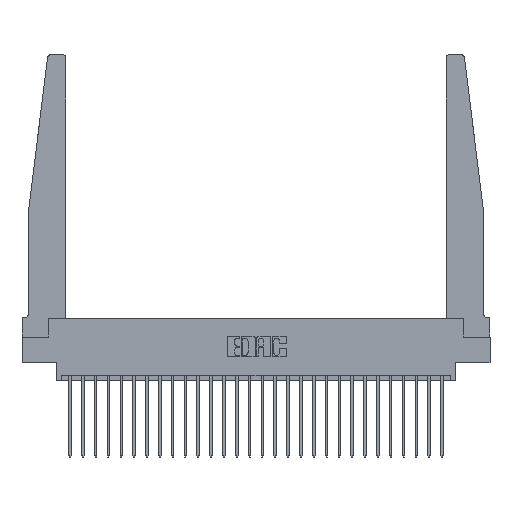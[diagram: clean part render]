
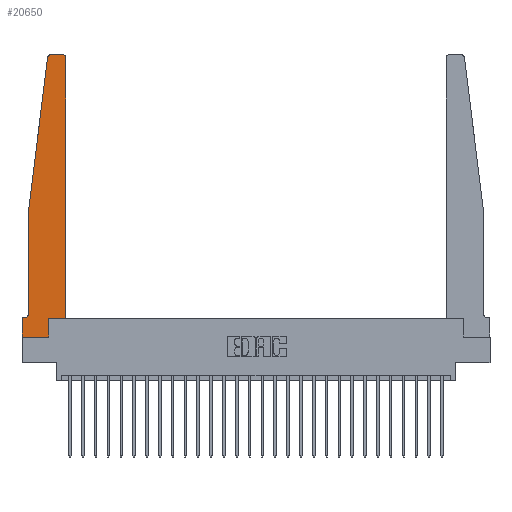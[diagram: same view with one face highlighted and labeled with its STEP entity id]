
A CAD part, top view. The second image highlights one B-rep face of the part: STEP entity #20650.
In plain terms, the highlighted planar face has unit normal (0, 0, 1).
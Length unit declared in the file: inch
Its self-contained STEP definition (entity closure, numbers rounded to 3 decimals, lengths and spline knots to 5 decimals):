
#593 = CARTESIAN_POINT ( 'NONE',  ( 0.395, 2.75, 0.37 ) ) ;
#656 = CARTESIAN_POINT ( 'NONE',  ( 0.2605, 0.18, 0.37 ) ) ;
#1507 = EDGE_LOOP ( 'NONE', ( #20498, #9159, #24146, #10517, #12868, #6242, #23240, #23998, #9563, #15301, #3218, #22295 ) ) ;
#1535 = VERTEX_POINT ( 'NONE', #5491 ) ;
#1877 = CARTESIAN_POINT ( 'NONE',  ( 0.065, 1.25, 0.37 ) ) ;
#2134 = EDGE_CURVE ( 'NONE', #16130, #18768, #19901, .T. ) ;
#2393 = DIRECTION ( 'NONE',  ( -1., 0., 0. ) ) ;
#2417 = CARTESIAN_POINT ( 'NONE',  ( 0.2605, 0.18, 0.37 ) ) ;
#2565 = AXIS2_PLACEMENT_3D ( 'NONE', #11643, #25686, #13702 ) ;
#2702 = EDGE_CURVE ( 'NONE', #18005, #11768, #7835, .T. ) ;
#2938 = AXIS2_PLACEMENT_3D ( 'NONE', #18687, #6571, #20726 ) ;
#3218 = ORIENTED_EDGE ( 'NONE', *, *, #19255, .T. ) ;
#3712 = VECTOR ( 'NONE', #24651, 39.37008 ) ;
#3942 = DIRECTION ( 'NONE',  ( 0., -1., 0. ) ) ;
#4295 = LINE ( 'NONE', #1877, #14464 ) ;
#4503 = CIRCLE ( 'NONE', #8227, 0.03 ) ;
#5489 = EDGE_CURVE ( 'NONE', #10939, #11011, #11783, .T. ) ;
#5491 = CARTESIAN_POINT ( 'NONE',  ( 0., 0., 0.37 ) ) ;
#5632 = CARTESIAN_POINT ( 'NONE',  ( 0.2605, 0., 0.37 ) ) ;
#6242 = ORIENTED_EDGE ( 'NONE', *, *, #2134, .T. ) ;
#6341 = EDGE_CURVE ( 'NONE', #15862, #16130, #15531, .T. ) ;
#6571 = DIRECTION ( 'NONE',  ( 0., 0., -1. ) ) ;
#6700 = DIRECTION ( 'NONE',  ( 1., 0., 0. ) ) ;
#7031 = VERTEX_POINT ( 'NONE', #2417 ) ;
#7835 = LINE ( 'NONE', #14583, #19243 ) ;
#8184 = AXIS2_PLACEMENT_3D ( 'NONE', #9942, #24029, #11977 ) ;
#8227 = AXIS2_PLACEMENT_3D ( 'NONE', #9074, #23188, #11116 ) ;
#8723 = LINE ( 'NONE', #24574, #23569 ) ;
#9074 = CARTESIAN_POINT ( 'NONE',  ( 0.27653, 2.72, 0.37 ) ) ;
#9159 = ORIENTED_EDGE ( 'NONE', *, *, #22400, .T. ) ;
#9563 = ORIENTED_EDGE ( 'NONE', *, *, #18704, .T. ) ;
#9791 = VECTOR ( 'NONE', #16907, 39.37008 ) ;
#9815 = CARTESIAN_POINT ( 'NONE',  ( 0.015, 0.1875, 0.37 ) ) ;
#9942 = CARTESIAN_POINT ( 'NONE',  ( 0.395, 2.72, 0.37 ) ) ;
#10312 = CARTESIAN_POINT ( 'NONE',  ( 0.24675, 2.72367, 0.37 ) ) ;
#10355 = DIRECTION ( 'NONE',  ( -1., 0., 0. ) ) ;
#10447 = VERTEX_POINT ( 'NONE', #5632 ) ;
#10517 = ORIENTED_EDGE ( 'NONE', *, *, #16203, .T. ) ;
#10580 = CARTESIAN_POINT ( 'NONE',  ( 0.425, 0.18, 0.37 ) ) ;
#10719 = CARTESIAN_POINT ( 'NONE',  ( 0.425, 0.18, 0.37 ) ) ;
#10727 = EDGE_CURVE ( 'NONE', #18768, #1535, #8723, .T. ) ;
#10743 = VECTOR ( 'NONE', #6700, 39.37008 ) ;
#10939 = VERTEX_POINT ( 'NONE', #10312 ) ;
#11011 = VERTEX_POINT ( 'NONE', #14552 ) ;
#11116 = DIRECTION ( 'NONE',  ( 1., 0., 0. ) ) ;
#11643 = CARTESIAN_POINT ( 'NONE',  ( 0., 0.1875, 0.37 ) ) ;
#11666 = DIRECTION ( 'NONE',  ( -0.122, -0.992, 0. ) ) ;
#11768 = VERTEX_POINT ( 'NONE', #12862 ) ;
#11783 = LINE ( 'NONE', #13730, #21899 ) ;
#11867 = EDGE_CURVE ( 'NONE', #7031, #25338, #25058, .T. ) ;
#11977 = DIRECTION ( 'NONE',  ( 1., 0., 0. ) ) ;
#12405 = CARTESIAN_POINT ( 'NONE',  ( 0.065, 0.1875, 0.37 ) ) ;
#12847 = VERTEX_POINT ( 'NONE', #16609 ) ;
#12862 = CARTESIAN_POINT ( 'NONE',  ( 0.27653, 2.75, 0.37 ) ) ;
#12868 = ORIENTED_EDGE ( 'NONE', *, *, #6341, .T. ) ;
#13219 = DIRECTION ( 'NONE',  ( 1., 0., 0. ) ) ;
#13702 = DIRECTION ( 'NONE',  ( 1., 0., 0. ) ) ;
#13730 = CARTESIAN_POINT ( 'NONE',  ( 0.065, 1.25, 0.37 ) ) ;
#13872 = CIRCLE ( 'NONE', #8184, 0.03 ) ;
#14464 = VECTOR ( 'NONE', #3942, 39.37008 ) ;
#14494 = EDGE_CURVE ( 'NONE', #1535, #10447, #24881, .T. ) ;
#14531 = VECTOR ( 'NONE', #10355, 39.37008 ) ;
#14552 = CARTESIAN_POINT ( 'NONE',  ( 0.065, 1.25, 0.37 ) ) ;
#14576 = DIRECTION ( 'NONE',  ( 0., -1., 0. ) ) ;
#14583 = CARTESIAN_POINT ( 'NONE',  ( 0.25, 2.75, 0.37 ) ) ;
#15301 = ORIENTED_EDGE ( 'NONE', *, *, #11867, .T. ) ;
#15531 = CIRCLE ( 'NONE', #2938, 0.05 ) ;
#15711 = FACE_OUTER_BOUND ( 'NONE', #1507, .T. ) ;
#15862 = VERTEX_POINT ( 'NONE', #25045 ) ;
#16130 = VERTEX_POINT ( 'NONE', #9815 ) ;
#16203 = EDGE_CURVE ( 'NONE', #11011, #15862, #4295, .T. ) ;
#16609 = CARTESIAN_POINT ( 'NONE',  ( 0.425, 2.72, 0.37 ) ) ;
#16907 = DIRECTION ( 'NONE',  ( 0., 1., 0. ) ) ;
#17649 = PLANE ( 'NONE',  #2565 ) ;
#18005 = VERTEX_POINT ( 'NONE', #593 ) ;
#18687 = CARTESIAN_POINT ( 'NONE',  ( 0.015, 0.2375, 0.37 ) ) ;
#18704 = EDGE_CURVE ( 'NONE', #10447, #7031, #25824, .T. ) ;
#18768 = VERTEX_POINT ( 'NONE', #23032 ) ;
#19131 = VECTOR ( 'NONE', #13219, 39.37008 ) ;
#19243 = VECTOR ( 'NONE', #2393, 39.37008 ) ;
#19254 = LINE ( 'NONE', #10580, #3712 ) ;
#19255 = EDGE_CURVE ( 'NONE', #25338, #12847, #19254, .T. ) ;
#19750 = EDGE_CURVE ( 'NONE', #12847, #18005, #13872, .T. ) ;
#19901 = LINE ( 'NONE', #12405, #14531 ) ;
#20498 = ORIENTED_EDGE ( 'NONE', *, *, #2702, .T. ) ;
#20650 = ADVANCED_FACE ( 'NONE', ( #15711 ), #17649, .T. ) ;
#20726 = DIRECTION ( 'NONE',  ( -1., 0., 0. ) ) ;
#20847 = CARTESIAN_POINT ( 'NONE',  ( 0., 0., 0.37 ) ) ;
#21899 = VECTOR ( 'NONE', #11666, 39.37008 ) ;
#22295 = ORIENTED_EDGE ( 'NONE', *, *, #19750, .T. ) ;
#22400 = EDGE_CURVE ( 'NONE', #11768, #10939, #4503, .T. ) ;
#23032 = CARTESIAN_POINT ( 'NONE',  ( 0., 0.1875, 0.37 ) ) ;
#23188 = DIRECTION ( 'NONE',  ( 0., 0., 1. ) ) ;
#23227 = CARTESIAN_POINT ( 'NONE',  ( 0.425, 0.18, 0.37 ) ) ;
#23240 = ORIENTED_EDGE ( 'NONE', *, *, #10727, .T. ) ;
#23569 = VECTOR ( 'NONE', #14576, 39.37008 ) ;
#23998 = ORIENTED_EDGE ( 'NONE', *, *, #14494, .T. ) ;
#24029 = DIRECTION ( 'NONE',  ( 0., 0., 1. ) ) ;
#24146 = ORIENTED_EDGE ( 'NONE', *, *, #5489, .T. ) ;
#24574 = CARTESIAN_POINT ( 'NONE',  ( 0., 0., 0.37 ) ) ;
#24651 = DIRECTION ( 'NONE',  ( 0., 1., 0. ) ) ;
#24881 = LINE ( 'NONE', #20847, #10743 ) ;
#25045 = CARTESIAN_POINT ( 'NONE',  ( 0.065, 0.2375, 0.37 ) ) ;
#25058 = LINE ( 'NONE', #23227, #19131 ) ;
#25338 = VERTEX_POINT ( 'NONE', #10719 ) ;
#25686 = DIRECTION ( 'NONE',  ( 0., 0., 1. ) ) ;
#25824 = LINE ( 'NONE', #656, #9791 ) ;
